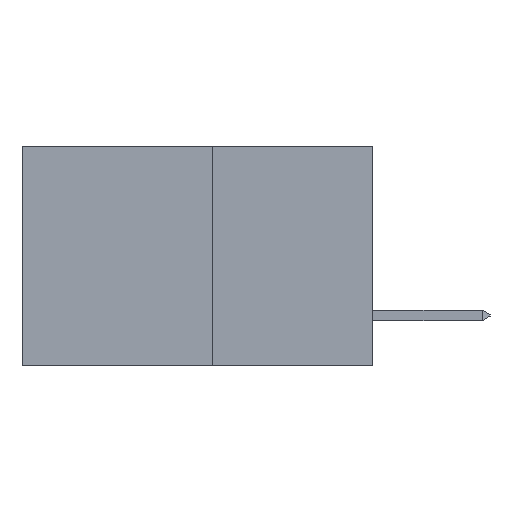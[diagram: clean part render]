
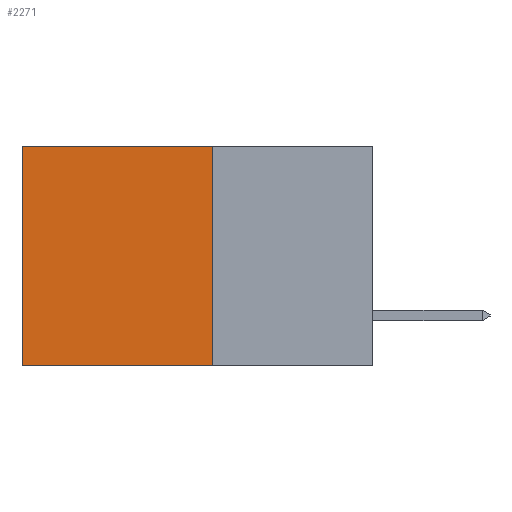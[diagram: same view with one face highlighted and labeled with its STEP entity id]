
A CAD part, left-side view. The second image highlights one B-rep face of the part: STEP entity #2271.
In plain terms, the highlighted planar face has unit normal (-1, 0, 0).
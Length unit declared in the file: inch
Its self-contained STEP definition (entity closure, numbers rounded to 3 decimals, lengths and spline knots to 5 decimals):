
#54 = LINE ( 'NONE', #5151, #2451 ) ;
#72 = VECTOR ( 'NONE', #10249, 39.37008 ) ;
#403 = LINE ( 'NONE', #7330, #8508 ) ;
#1075 = DIRECTION ( 'NONE',  ( 1., 0., 0. ) ) ;
#1325 = EDGE_CURVE ( 'NONE', #8379, #7988, #6557, .T. ) ;
#1811 = CARTESIAN_POINT ( 'NONE',  ( 0.277, 0.27, 0. ) ) ;
#2271 = ADVANCED_FACE ( 'NONE', ( #3310 ), #4074, .F. ) ;
#2451 = VECTOR ( 'NONE', #2688, 39.37008 ) ;
#2594 = EDGE_CURVE ( 'NONE', #4532, #2763, #403, .T. ) ;
#2688 = DIRECTION ( 'NONE',  ( 0., 1., 0. ) ) ;
#2763 = VERTEX_POINT ( 'NONE', #6619 ) ;
#3173 = ORIENTED_EDGE ( 'NONE', *, *, #1325, .F. ) ;
#3310 = FACE_OUTER_BOUND ( 'NONE', #9209, .T. ) ;
#4071 = CARTESIAN_POINT ( 'NONE',  ( 0.277, 0.27, -0.37 ) ) ;
#4074 = PLANE ( 'NONE',  #7016 ) ;
#4532 = VERTEX_POINT ( 'NONE', #7085 ) ;
#5015 = VECTOR ( 'NONE', #8542, 39.37008 ) ;
#5151 = CARTESIAN_POINT ( 'NONE',  ( 0.277, 0.27, -0.37 ) ) ;
#5233 = ORIENTED_EDGE ( 'NONE', *, *, #6617, .T. ) ;
#5487 = LINE ( 'NONE', #8710, #5015 ) ;
#5810 = EDGE_CURVE ( 'NONE', #7988, #2763, #54, .T. ) ;
#5931 = DIRECTION ( 'NONE',  ( 0., 0., -1. ) ) ;
#6359 = DIRECTION ( 'NONE',  ( 0., 0., -1. ) ) ;
#6557 = LINE ( 'NONE', #9499, #72 ) ;
#6617 = EDGE_CURVE ( 'NONE', #8379, #4532, #5487, .T. ) ;
#6619 = CARTESIAN_POINT ( 'NONE',  ( 0.277, 0.59, -0.37 ) ) ;
#6984 = ORIENTED_EDGE ( 'NONE', *, *, #2594, .T. ) ;
#7016 = AXIS2_PLACEMENT_3D ( 'NONE', #4071, #1075, #5931 ) ;
#7085 = CARTESIAN_POINT ( 'NONE',  ( 0.277, 0.59, 0. ) ) ;
#7330 = CARTESIAN_POINT ( 'NONE',  ( 0.277, 0.59, -0.37 ) ) ;
#7988 = VERTEX_POINT ( 'NONE', #8325 ) ;
#8325 = CARTESIAN_POINT ( 'NONE',  ( 0.277, 0.27, -0.37 ) ) ;
#8379 = VERTEX_POINT ( 'NONE', #1811 ) ;
#8508 = VECTOR ( 'NONE', #6359, 39.37008 ) ;
#8542 = DIRECTION ( 'NONE',  ( 0., 1., 0. ) ) ;
#8710 = CARTESIAN_POINT ( 'NONE',  ( 0.277, 0.27, 0. ) ) ;
#8977 = ORIENTED_EDGE ( 'NONE', *, *, #5810, .F. ) ;
#9209 = EDGE_LOOP ( 'NONE', ( #6984, #8977, #3173, #5233 ) ) ;
#9499 = CARTESIAN_POINT ( 'NONE',  ( 0.277, 0.27, -0.37 ) ) ;
#10249 = DIRECTION ( 'NONE',  ( 0., 0., -1. ) ) ;
